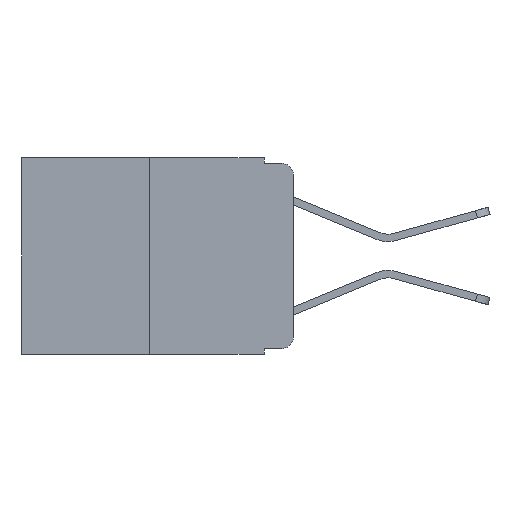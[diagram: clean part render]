
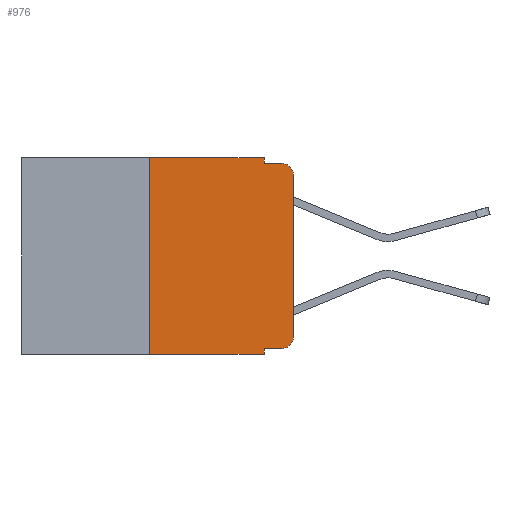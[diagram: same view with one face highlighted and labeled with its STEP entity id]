
A CAD part, left-side view. The second image highlights one B-rep face of the part: STEP entity #976.
In plain terms, the highlighted planar face has unit normal (-1, 0, 0).
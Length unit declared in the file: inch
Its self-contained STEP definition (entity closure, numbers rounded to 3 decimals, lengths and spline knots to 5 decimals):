
#156 = CARTESIAN_POINT ( 'NONE',  ( 0., 0.02, -0.333 ) ) ;
#286 = DIRECTION ( 'NONE',  ( 0., 0., 1. ) ) ;
#341 = VERTEX_POINT ( 'NONE', #14901 ) ;
#393 = VERTEX_POINT ( 'NONE', #12034 ) ;
#711 = CARTESIAN_POINT ( 'NONE',  ( 0., 0.473, 0. ) ) ;
#801 = EDGE_CURVE ( 'NONE', #12221, #4170, #6081, .T. ) ;
#821 = DIRECTION ( 'NONE',  ( 0., 0., 1. ) ) ;
#935 = ORIENTED_EDGE ( 'NONE', *, *, #801, .F. ) ;
#976 = ADVANCED_FACE ( 'NONE', ( #14481 ), #4069, .F. ) ;
#1214 = DIRECTION ( 'NONE',  ( -1., 0., 0. ) ) ;
#1914 = EDGE_CURVE ( 'NONE', #7354, #13939, #19471, .T. ) ;
#2468 = VERTEX_POINT ( 'NONE', #13283 ) ;
#2854 = CARTESIAN_POINT ( 'NONE',  ( 0., 0.25, -0.343 ) ) ;
#2949 = LINE ( 'NONE', #9807, #10854 ) ;
#3203 = ORIENTED_EDGE ( 'NONE', *, *, #7894, .F. ) ;
#3322 = CARTESIAN_POINT ( 'NONE',  ( 0., 0.051, 0. ) ) ;
#3326 = DIRECTION ( 'NONE',  ( -1., 0., 0. ) ) ;
#3577 = CARTESIAN_POINT ( 'NONE',  ( 0., 0.25, 0. ) ) ;
#3976 = EDGE_LOOP ( 'NONE', ( #13036, #4639, #8592, #5163, #3203, #935, #7597, #11232, #18410, #16255 ) ) ;
#3982 = VECTOR ( 'NONE', #9188, 39.37008 ) ;
#4013 = CARTESIAN_POINT ( 'NONE',  ( 0., 0.051, -0.01 ) ) ;
#4069 = PLANE ( 'NONE',  #4479 ) ;
#4164 = EDGE_CURVE ( 'NONE', #13939, #341, #2949, .T. ) ;
#4170 = VERTEX_POINT ( 'NONE', #5167 ) ;
#4479 = AXIS2_PLACEMENT_3D ( 'NONE', #711, #16413, #7238 ) ;
#4639 = ORIENTED_EDGE ( 'NONE', *, *, #5241, .T. ) ;
#4837 = VERTEX_POINT ( 'NONE', #156 ) ;
#5048 = DIRECTION ( 'NONE',  ( 0., -1., 0. ) ) ;
#5163 = ORIENTED_EDGE ( 'NONE', *, *, #1914, .F. ) ;
#5167 = CARTESIAN_POINT ( 'NONE',  ( 0., 0.25, 0. ) ) ;
#5241 = EDGE_CURVE ( 'NONE', #15787, #341, #8886, .T. ) ;
#5619 = LINE ( 'NONE', #17369, #16910 ) ;
#5725 = CARTESIAN_POINT ( 'NONE',  ( 0., 0., 0. ) ) ;
#6081 = LINE ( 'NONE', #3577, #14265 ) ;
#6287 = EDGE_CURVE ( 'NONE', #393, #15787, #18858, .T. ) ;
#7238 = DIRECTION ( 'NONE',  ( 0., 0., -1. ) ) ;
#7354 = VERTEX_POINT ( 'NONE', #8500 ) ;
#7384 = VERTEX_POINT ( 'NONE', #13129 ) ;
#7597 = ORIENTED_EDGE ( 'NONE', *, *, #18264, .T. ) ;
#7894 = EDGE_CURVE ( 'NONE', #4170, #7354, #5619, .T. ) ;
#8123 = LINE ( 'NONE', #19725, #19825 ) ;
#8201 = LINE ( 'NONE', #18334, #3982 ) ;
#8251 = VECTOR ( 'NONE', #12704, 39.37008 ) ;
#8500 = CARTESIAN_POINT ( 'NONE',  ( 0., 0.051, 0. ) ) ;
#8592 = ORIENTED_EDGE ( 'NONE', *, *, #4164, .F. ) ;
#8877 = AXIS2_PLACEMENT_3D ( 'NONE', #10791, #1214, #12348 ) ;
#8886 = CIRCLE ( 'NONE', #8877, 0.02 ) ;
#9188 = DIRECTION ( 'NONE',  ( 0., -1., 0. ) ) ;
#9807 = CARTESIAN_POINT ( 'NONE',  ( 0., 0.051, -0.01 ) ) ;
#10262 = VECTOR ( 'NONE', #821, 39.37008 ) ;
#10578 = VECTOR ( 'NONE', #13950, 39.37008 ) ;
#10600 = DIRECTION ( 'NONE',  ( 0., 0., -1. ) ) ;
#10791 = CARTESIAN_POINT ( 'NONE',  ( 0., 0.02, -0.03 ) ) ;
#10854 = VECTOR ( 'NONE', #12767, 39.37008 ) ;
#11232 = ORIENTED_EDGE ( 'NONE', *, *, #20032, .F. ) ;
#12034 = CARTESIAN_POINT ( 'NONE',  ( 0., 0., -0.313 ) ) ;
#12221 = VERTEX_POINT ( 'NONE', #2854 ) ;
#12348 = DIRECTION ( 'NONE',  ( 0., 0., -1. ) ) ;
#12469 = CARTESIAN_POINT ( 'NONE',  ( 0., 0.051, -0.333 ) ) ;
#12704 = DIRECTION ( 'NONE',  ( 0., 0., -1. ) ) ;
#12712 = CARTESIAN_POINT ( 'NONE',  ( 0., 0.02, -0.313 ) ) ;
#12767 = DIRECTION ( 'NONE',  ( 0., -1., 0. ) ) ;
#13036 = ORIENTED_EDGE ( 'NONE', *, *, #6287, .T. ) ;
#13129 = CARTESIAN_POINT ( 'NONE',  ( 0., 0.051, -0.343 ) ) ;
#13283 = CARTESIAN_POINT ( 'NONE',  ( 0., 0.051, -0.333 ) ) ;
#13939 = VERTEX_POINT ( 'NONE', #4013 ) ;
#13950 = DIRECTION ( 'NONE',  ( 0., -1., 0. ) ) ;
#14203 = DIRECTION ( 'NONE',  ( 0., 0., -1. ) ) ;
#14243 = CARTESIAN_POINT ( 'NONE',  ( 0., 0., -0.03 ) ) ;
#14265 = VECTOR ( 'NONE', #286, 39.37008 ) ;
#14481 = FACE_OUTER_BOUND ( 'NONE', #3976, .T. ) ;
#14901 = CARTESIAN_POINT ( 'NONE',  ( 0., 0.02, -0.01 ) ) ;
#15787 = VERTEX_POINT ( 'NONE', #14243 ) ;
#16255 = ORIENTED_EDGE ( 'NONE', *, *, #16974, .T. ) ;
#16413 = DIRECTION ( 'NONE',  ( 1., 0., 0. ) ) ;
#16910 = VECTOR ( 'NONE', #5048, 39.37008 ) ;
#16974 = EDGE_CURVE ( 'NONE', #4837, #393, #17778, .T. ) ;
#17369 = CARTESIAN_POINT ( 'NONE',  ( 0., 0.473, 0. ) ) ;
#17778 = CIRCLE ( 'NONE', #17861, 0.02 ) ;
#17861 = AXIS2_PLACEMENT_3D ( 'NONE', #12712, #3326, #14203 ) ;
#18264 = EDGE_CURVE ( 'NONE', #12221, #7384, #8201, .T. ) ;
#18334 = CARTESIAN_POINT ( 'NONE',  ( 0., 0.473, -0.343 ) ) ;
#18410 = ORIENTED_EDGE ( 'NONE', *, *, #19009, .T. ) ;
#18674 = LINE ( 'NONE', #12469, #10578 ) ;
#18858 = LINE ( 'NONE', #5725, #10262 ) ;
#19009 = EDGE_CURVE ( 'NONE', #2468, #4837, #18674, .T. ) ;
#19471 = LINE ( 'NONE', #3322, #8251 ) ;
#19725 = CARTESIAN_POINT ( 'NONE',  ( 0., 0.051, 0. ) ) ;
#19825 = VECTOR ( 'NONE', #10600, 39.37008 ) ;
#20032 = EDGE_CURVE ( 'NONE', #2468, #7384, #8123, .T. ) ;
